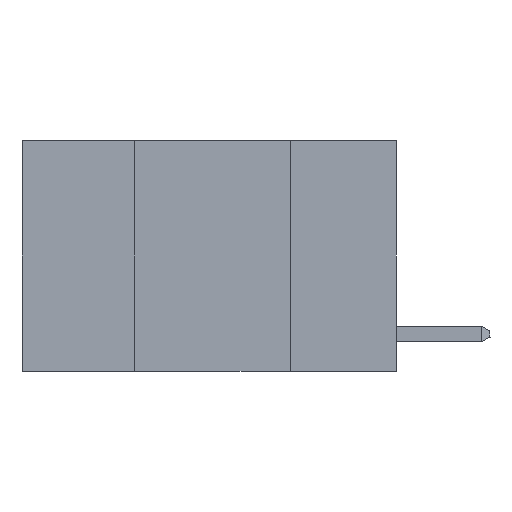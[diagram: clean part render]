
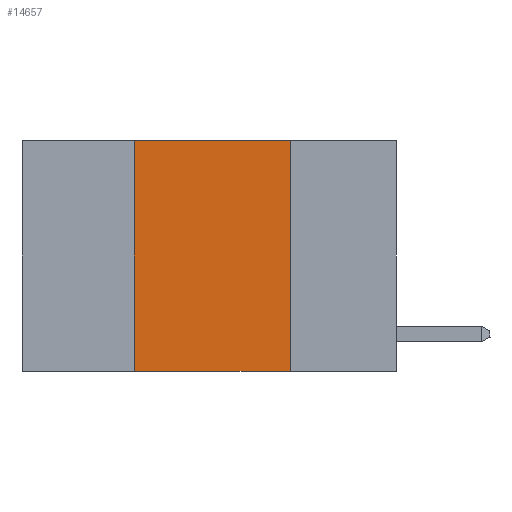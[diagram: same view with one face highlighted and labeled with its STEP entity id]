
A CAD part, left-side view. The second image highlights one B-rep face of the part: STEP entity #14657.
In plain terms, the highlighted planar face has unit normal (-1, 0, 0).
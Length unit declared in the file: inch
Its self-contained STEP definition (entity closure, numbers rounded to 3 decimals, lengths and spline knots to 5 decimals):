
#503 = VERTEX_POINT ( 'NONE', #1157 ) ;
#966 = EDGE_CURVE ( 'NONE', #503, #3376, #3109, .T. ) ;
#1157 = CARTESIAN_POINT ( 'NONE',  ( 0., 0.17, 0. ) ) ;
#1805 = ORIENTED_EDGE ( 'NONE', *, *, #20764, .T. ) ;
#2341 = DIRECTION ( 'NONE',  ( 0., 0., 1. ) ) ;
#3002 = CARTESIAN_POINT ( 'NONE',  ( 0., 0.17, 0. ) ) ;
#3109 = LINE ( 'NONE', #3002, #10491 ) ;
#3376 = VERTEX_POINT ( 'NONE', #7553 ) ;
#3701 = CARTESIAN_POINT ( 'NONE',  ( 0., 0.42, 0. ) ) ;
#3827 = VERTEX_POINT ( 'NONE', #5235 ) ;
#5113 = CARTESIAN_POINT ( 'NONE',  ( 0., 0.42, -0.37 ) ) ;
#5235 = CARTESIAN_POINT ( 'NONE',  ( 0., 0.42, 0. ) ) ;
#7184 = FACE_OUTER_BOUND ( 'NONE', #9168, .T. ) ;
#7553 = CARTESIAN_POINT ( 'NONE',  ( 0., 0.17, -0.37 ) ) ;
#9168 = EDGE_LOOP ( 'NONE', ( #18538, #15436, #15996, #1805 ) ) ;
#9211 = DIRECTION ( 'NONE',  ( 0., 0., -1. ) ) ;
#9433 = EDGE_CURVE ( 'NONE', #3827, #503, #16783, .T. ) ;
#10027 = VECTOR ( 'NONE', #10168, 39.37008 ) ;
#10168 = DIRECTION ( 'NONE',  ( 0., -1., 0. ) ) ;
#10491 = VECTOR ( 'NONE', #9211, 39.37008 ) ;
#11021 = CARTESIAN_POINT ( 'NONE',  ( 0., 0.6, -0.37 ) ) ;
#11870 = VECTOR ( 'NONE', #12820, 39.37008 ) ;
#12820 = DIRECTION ( 'NONE',  ( 0., -1., 0. ) ) ;
#13064 = EDGE_CURVE ( 'NONE', #15197, #3827, #16430, .T. ) ;
#13842 = DIRECTION ( 'NONE',  ( 0., 0., -1. ) ) ;
#14428 = VECTOR ( 'NONE', #2341, 39.37008 ) ;
#14657 = ADVANCED_FACE ( 'NONE', ( #7184 ), #18478, .F. ) ;
#15197 = VERTEX_POINT ( 'NONE', #5113 ) ;
#15436 = ORIENTED_EDGE ( 'NONE', *, *, #9433, .F. ) ;
#15996 = ORIENTED_EDGE ( 'NONE', *, *, #13064, .F. ) ;
#16430 = LINE ( 'NONE', #3701, #14428 ) ;
#16473 = CARTESIAN_POINT ( 'NONE',  ( 0., 0.6, 0. ) ) ;
#16660 = CARTESIAN_POINT ( 'NONE',  ( 0., 0.6, 0. ) ) ;
#16783 = LINE ( 'NONE', #16473, #10027 ) ;
#17438 = LINE ( 'NONE', #11021, #11870 ) ;
#18478 = PLANE ( 'NONE',  #19562 ) ;
#18538 = ORIENTED_EDGE ( 'NONE', *, *, #966, .F. ) ;
#19562 = AXIS2_PLACEMENT_3D ( 'NONE', #16660, #19969, #13842 ) ;
#19969 = DIRECTION ( 'NONE',  ( 1., 0., 0. ) ) ;
#20764 = EDGE_CURVE ( 'NONE', #15197, #3376, #17438, .T. ) ;
